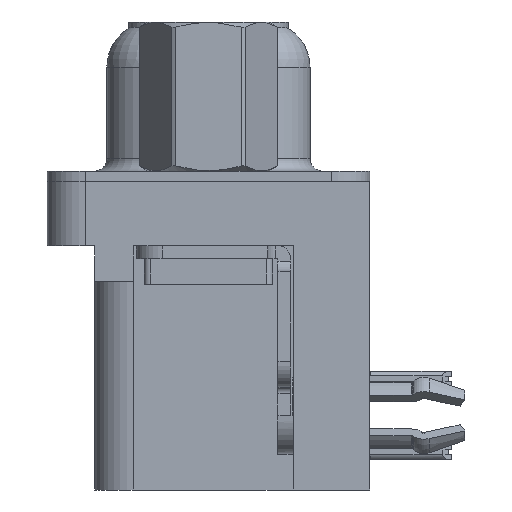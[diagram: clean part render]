
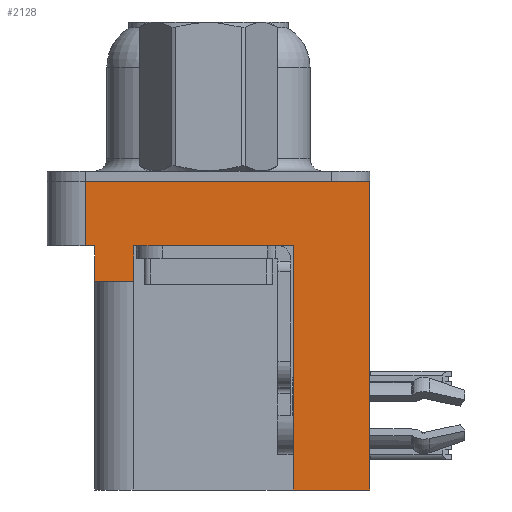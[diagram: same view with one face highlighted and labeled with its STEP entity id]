
A CAD part, left-side view. The second image highlights one B-rep face of the part: STEP entity #2128.
In plain terms, the highlighted planar face has unit normal (-1, 0, 0).
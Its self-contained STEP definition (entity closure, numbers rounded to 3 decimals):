
#74 = VERTEX_POINT ( 'NONE', #26625 ) ;
#243 = CARTESIAN_POINT ( 'NONE',  ( -2.91, 4.425, -2.5 ) ) ;
#409 = CARTESIAN_POINT ( 'NONE',  ( -2.91, 2.895, -2.5 ) ) ;
#559 = LINE ( 'NONE', #13311, #18463 ) ;
#1235 = DIRECTION ( 'NONE',  ( 0., 0., 1. ) ) ;
#1637 = VERTEX_POINT ( 'NONE', #28007 ) ;
#2128 = ADVANCED_FACE ( 'NONE', ( #22654 ), #18167, .T. ) ;
#2349 = ORIENTED_EDGE ( 'NONE', *, *, #29322, .F. ) ;
#4106 = DIRECTION ( 'NONE',  ( -1., 0., 0. ) ) ;
#4541 = EDGE_CURVE ( 'NONE', #18591, #12421, #13682, .T. ) ;
#5492 = LINE ( 'NONE', #14017, #29568 ) ;
#5975 = VECTOR ( 'NONE', #12817, 1000. ) ;
#6934 = VECTOR ( 'NONE', #13363, 1000. ) ;
#7006 = LINE ( 'NONE', #15029, #17923 ) ;
#7126 = ORIENTED_EDGE ( 'NONE', *, *, #19135, .F. ) ;
#7255 = EDGE_CURVE ( 'NONE', #9749, #29419, #7006, .T. ) ;
#7421 = ORIENTED_EDGE ( 'NONE', *, *, #7255, .T. ) ;
#7506 = AXIS2_PLACEMENT_3D ( 'NONE', #18059, #4106, #11162 ) ;
#7559 = ORIENTED_EDGE ( 'NONE', *, *, #11837, .T. ) ;
#8383 = VECTOR ( 'NONE', #1235, 1000. ) ;
#8399 = LINE ( 'NONE', #11742, #19726 ) ;
#8409 = CARTESIAN_POINT ( 'NONE',  ( -2.91, -6.275, -2.5 ) ) ;
#8688 = ORIENTED_EDGE ( 'NONE', *, *, #17244, .F. ) ;
#8741 = LINE ( 'NONE', #27031, #8383 ) ;
#9582 = VECTOR ( 'NONE', #12038, 1000. ) ;
#9749 = VERTEX_POINT ( 'NONE', #17603 ) ;
#10384 = VERTEX_POINT ( 'NONE', #13831 ) ;
#10579 = VECTOR ( 'NONE', #15057, 1000. ) ;
#11162 = DIRECTION ( 'NONE',  ( 0., 0., 1. ) ) ;
#11742 = CARTESIAN_POINT ( 'NONE',  ( -2.91, -3.295, -12. ) ) ;
#11837 = EDGE_CURVE ( 'NONE', #1637, #21379, #26942, .T. ) ;
#12036 = DIRECTION ( 'NONE',  ( 0., 0., 1. ) ) ;
#12038 = DIRECTION ( 'NONE',  ( 0., 1., 0. ) ) ;
#12421 = VERTEX_POINT ( 'NONE', #23093 ) ;
#12817 = DIRECTION ( 'NONE',  ( 0., -1., 0. ) ) ;
#13140 = LINE ( 'NONE', #27302, #6934 ) ;
#13311 = CARTESIAN_POINT ( 'NONE',  ( -2.91, 4.425, -3.9 ) ) ;
#13363 = DIRECTION ( 'NONE',  ( 0., -1., 0. ) ) ;
#13682 = LINE ( 'NONE', #8409, #5975 ) ;
#13831 = CARTESIAN_POINT ( 'NONE',  ( -2.91, 4.425, -3.9 ) ) ;
#14017 = CARTESIAN_POINT ( 'NONE',  ( -2.91, 4.425, -3.9 ) ) ;
#14964 = CARTESIAN_POINT ( 'NONE',  ( -2.91, 2.895, -3.9 ) ) ;
#15029 = CARTESIAN_POINT ( 'NONE',  ( -2.91, -6.275, -2.5 ) ) ;
#15057 = DIRECTION ( 'NONE',  ( 0., 0., 1. ) ) ;
#15418 = DIRECTION ( 'NONE',  ( 0., 0., 1. ) ) ;
#16100 = ORIENTED_EDGE ( 'NONE', *, *, #28803, .F. ) ;
#16548 = DIRECTION ( 'NONE',  ( 0., 0., 1. ) ) ;
#17112 = VECTOR ( 'NONE', #15418, 1000. ) ;
#17244 = EDGE_CURVE ( 'NONE', #1637, #74, #28194, .T. ) ;
#17276 = VERTEX_POINT ( 'NONE', #14964 ) ;
#17497 = LINE ( 'NONE', #27046, #10579 ) ;
#17603 = CARTESIAN_POINT ( 'NONE',  ( -2.91, 4.775, -2.5 ) ) ;
#17923 = VECTOR ( 'NONE', #19698, 1000. ) ;
#18059 = CARTESIAN_POINT ( 'NONE',  ( -2.91, -6.275, -2.5 ) ) ;
#18167 = PLANE ( 'NONE',  #7506 ) ;
#18463 = VECTOR ( 'NONE', #20321, 1000. ) ;
#18589 = CARTESIAN_POINT ( 'NONE',  ( -2.91, -6.275, 0. ) ) ;
#18591 = VERTEX_POINT ( 'NONE', #409 ) ;
#19135 = EDGE_CURVE ( 'NONE', #9749, #21382, #8741, .T. ) ;
#19698 = DIRECTION ( 'NONE',  ( 0., -1., 0. ) ) ;
#19726 = VECTOR ( 'NONE', #12036, 1000. ) ;
#20321 = DIRECTION ( 'NONE',  ( 0., 1., 0. ) ) ;
#20485 = CARTESIAN_POINT ( 'NONE',  ( -2.91, -6.275, -2.5 ) ) ;
#20605 = EDGE_CURVE ( 'NONE', #17276, #18591, #17497, .T. ) ;
#20924 = CARTESIAN_POINT ( 'NONE',  ( -2.91, 4.775, 0. ) ) ;
#21216 = ORIENTED_EDGE ( 'NONE', *, *, #30193, .F. ) ;
#21379 = VERTEX_POINT ( 'NONE', #18589 ) ;
#21382 = VERTEX_POINT ( 'NONE', #20924 ) ;
#22654 = FACE_OUTER_BOUND ( 'NONE', #25997, .T. ) ;
#23093 = CARTESIAN_POINT ( 'NONE',  ( -2.91, -3.295, -2.5 ) ) ;
#23099 = ORIENTED_EDGE ( 'NONE', *, *, #4541, .T. ) ;
#24294 = EDGE_CURVE ( 'NONE', #17276, #10384, #559, .T. ) ;
#25997 = EDGE_LOOP ( 'NONE', ( #21216, #7126, #7421, #16100, #26312, #29110, #23099, #2349, #8688, #7559 ) ) ;
#26312 = ORIENTED_EDGE ( 'NONE', *, *, #24294, .F. ) ;
#26625 = CARTESIAN_POINT ( 'NONE',  ( -2.91, -3.295, -12. ) ) ;
#26942 = LINE ( 'NONE', #20485, #17112 ) ;
#27031 = CARTESIAN_POINT ( 'NONE',  ( -2.91, 4.775, -2.5 ) ) ;
#27046 = CARTESIAN_POINT ( 'NONE',  ( -2.91, 2.895, -3.9 ) ) ;
#27302 = CARTESIAN_POINT ( 'NONE',  ( -2.91, -6.275, 0. ) ) ;
#28007 = CARTESIAN_POINT ( 'NONE',  ( -2.91, -6.275, -12. ) ) ;
#28194 = LINE ( 'NONE', #28418, #9582 ) ;
#28418 = CARTESIAN_POINT ( 'NONE',  ( -2.91, -3.295, -12. ) ) ;
#28803 = EDGE_CURVE ( 'NONE', #10384, #29419, #5492, .T. ) ;
#29110 = ORIENTED_EDGE ( 'NONE', *, *, #20605, .T. ) ;
#29322 = EDGE_CURVE ( 'NONE', #74, #12421, #8399, .T. ) ;
#29419 = VERTEX_POINT ( 'NONE', #243 ) ;
#29568 = VECTOR ( 'NONE', #16548, 1000. ) ;
#30193 = EDGE_CURVE ( 'NONE', #21382, #21379, #13140, .T. ) ;
